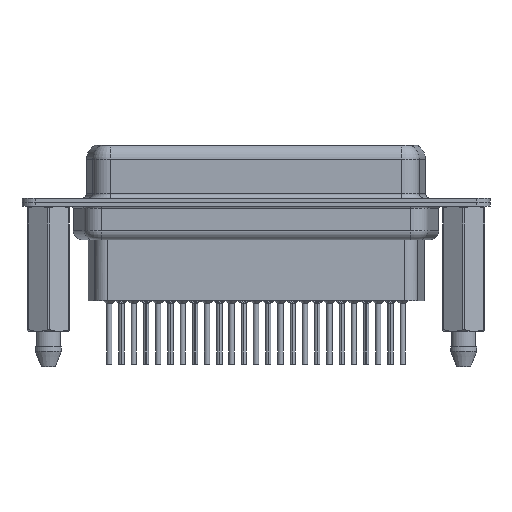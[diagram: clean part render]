
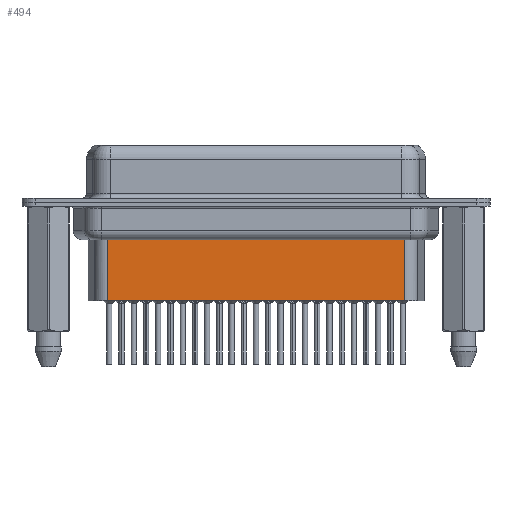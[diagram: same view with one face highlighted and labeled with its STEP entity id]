
A CAD part, front view. The second image highlights one B-rep face of the part: STEP entity #494.
In plain terms, the highlighted planar face has unit normal (0, -1, 0).
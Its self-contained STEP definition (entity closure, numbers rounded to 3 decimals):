
#494 = ADVANCED_FACE ( 'NONE', ( #15498 ), #18275, .T. ) ;
#1010 = CARTESIAN_POINT ( 'NONE',  ( 40.344, -3.5, -11.15 ) ) ;
#1319 = CARTESIAN_POINT ( 'NONE',  ( 6.706, -3.5, -3.1 ) ) ;
#4162 = EDGE_CURVE ( 'NONE', #9328, #15915, #28876, .T. ) ;
#4646 = EDGE_CURVE ( 'NONE', #11179, #14303, #21902, .T. ) ;
#5294 = ORIENTED_EDGE ( 'NONE', *, *, #22685, .F. ) ;
#5721 = ORIENTED_EDGE ( 'NONE', *, *, #16097, .T. ) ;
#5829 = CARTESIAN_POINT ( 'NONE',  ( 40.344, -3.5, -4.097 ) ) ;
#6331 = DIRECTION ( 'NONE',  ( 0., 0., -1. ) ) ;
#9292 = DIRECTION ( 'NONE',  ( 1., 0., 0. ) ) ;
#9328 = VERTEX_POINT ( 'NONE', #5829 ) ;
#10048 = EDGE_LOOP ( 'NONE', ( #11748, #5721, #24451, #5294 ) ) ;
#11179 = VERTEX_POINT ( 'NONE', #18193 ) ;
#11748 = ORIENTED_EDGE ( 'NONE', *, *, #4162, .F. ) ;
#12534 = CARTESIAN_POINT ( 'NONE',  ( 6.706, -3.5, -11.15 ) ) ;
#14303 = VERTEX_POINT ( 'NONE', #22695 ) ;
#15047 = DIRECTION ( 'NONE',  ( -1., 0., 0. ) ) ;
#15498 = FACE_OUTER_BOUND ( 'NONE', #10048, .T. ) ;
#15790 = DIRECTION ( 'NONE',  ( 0., -1., 0. ) ) ;
#15915 = VERTEX_POINT ( 'NONE', #1010 ) ;
#16097 = EDGE_CURVE ( 'NONE', #9328, #11179, #20255, .T. ) ;
#17744 = CARTESIAN_POINT ( 'NONE',  ( 6.459, -3.5, -4.097 ) ) ;
#18193 = CARTESIAN_POINT ( 'NONE',  ( 6.706, -3.5, -4.097 ) ) ;
#18275 = PLANE ( 'NONE',  #24756 ) ;
#19305 = CARTESIAN_POINT ( 'NONE',  ( 40.344, -3.5, -3.1 ) ) ;
#19405 = VECTOR ( 'NONE', #26741, 1000. ) ;
#19771 = VECTOR ( 'NONE', #6331, 1000. ) ;
#20255 = LINE ( 'NONE', #17744, #19405 ) ;
#20319 = VECTOR ( 'NONE', #23664, 1000. ) ;
#20345 = CARTESIAN_POINT ( 'NONE',  ( 6.706, -3.5, -3.1 ) ) ;
#21216 = VECTOR ( 'NONE', #15047, 1000. ) ;
#21902 = LINE ( 'NONE', #1319, #20319 ) ;
#22685 = EDGE_CURVE ( 'NONE', #15915, #14303, #28742, .T. ) ;
#22695 = CARTESIAN_POINT ( 'NONE',  ( 6.706, -3.5, -11.15 ) ) ;
#23664 = DIRECTION ( 'NONE',  ( 0., 0., -1. ) ) ;
#24451 = ORIENTED_EDGE ( 'NONE', *, *, #4646, .T. ) ;
#24756 = AXIS2_PLACEMENT_3D ( 'NONE', #20345, #15790, #9292 ) ;
#26741 = DIRECTION ( 'NONE',  ( -1., 0., 0. ) ) ;
#28742 = LINE ( 'NONE', #12534, #21216 ) ;
#28876 = LINE ( 'NONE', #19305, #19771 ) ;
